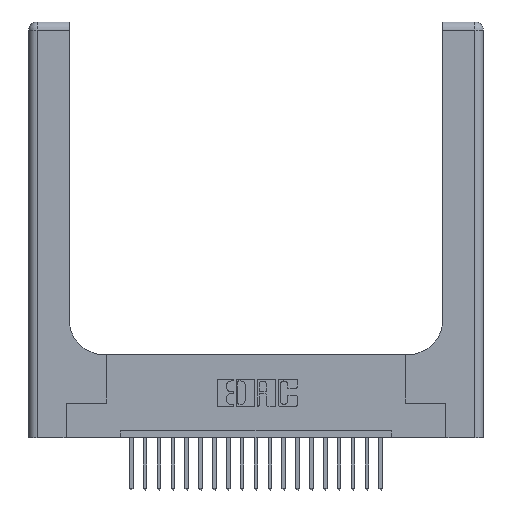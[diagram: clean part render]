
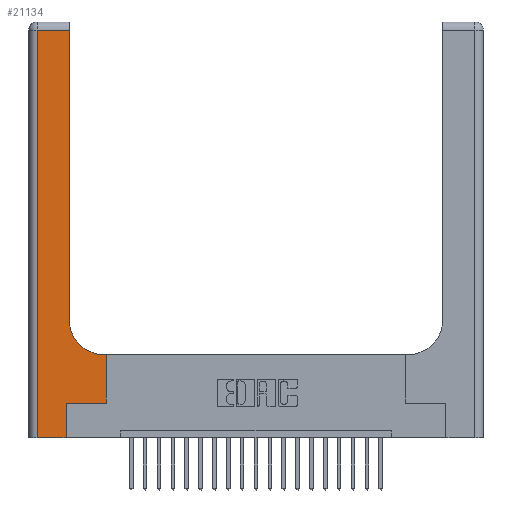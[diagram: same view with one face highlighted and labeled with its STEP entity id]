
A CAD part, top view. The second image highlights one B-rep face of the part: STEP entity #21134.
In plain terms, the highlighted planar face has unit normal (0, 0, 1).
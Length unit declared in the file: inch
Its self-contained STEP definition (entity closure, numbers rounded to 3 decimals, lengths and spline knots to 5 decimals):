
#349 = DIRECTION ( 'NONE',  ( 0., 1., 0. ) ) ;
#1554 = DIRECTION ( 'NONE',  ( 1., 0., 0. ) ) ;
#1664 = DIRECTION ( 'NONE',  ( 0., 0., -1. ) ) ;
#1735 = CARTESIAN_POINT ( 'NONE',  ( 0., 3., 0.37 ) ) ;
#2094 = LINE ( 'NONE', #3191, #18979 ) ;
#2331 = VERTEX_POINT ( 'NONE', #3034 ) ;
#2399 = DIRECTION ( 'NONE',  ( -1., 0., 0. ) ) ;
#2415 = CARTESIAN_POINT ( 'NONE',  ( 0.269, 0.25, 0.37 ) ) ;
#2566 = ORIENTED_EDGE ( 'NONE', *, *, #3840, .T. ) ;
#2600 = ORIENTED_EDGE ( 'NONE', *, *, #7431, .T. ) ;
#2825 = CARTESIAN_POINT ( 'NONE',  ( 0.5415, 0.6, 0.37 ) ) ;
#3034 = CARTESIAN_POINT ( 'NONE',  ( 0.5585, 0.25, 0.37 ) ) ;
#3191 = CARTESIAN_POINT ( 'NONE',  ( 0.5585, 0.25, 0.37 ) ) ;
#3840 = EDGE_CURVE ( 'NONE', #4231, #2331, #13804, .T. ) ;
#4231 = VERTEX_POINT ( 'NONE', #16587 ) ;
#4904 = DIRECTION ( 'NONE',  ( 0., -1., 0. ) ) ;
#4923 = VERTEX_POINT ( 'NONE', #15385 ) ;
#5019 = DIRECTION ( 'NONE',  ( -1., 0., 0. ) ) ;
#5157 = ORIENTED_EDGE ( 'NONE', *, *, #13256, .T. ) ;
#5191 = EDGE_LOOP ( 'NONE', ( #15216, #2600, #5157, #20965, #13100, #2566, #22404, #15001, #20932 ) ) ;
#6189 = LINE ( 'NONE', #8188, #12143 ) ;
#6477 = VECTOR ( 'NONE', #349, 39.37008 ) ;
#7431 = EDGE_CURVE ( 'NONE', #22213, #4923, #16874, .T. ) ;
#7611 = CARTESIAN_POINT ( 'NONE',  ( 0.2915, 0.6, 0.37 ) ) ;
#7626 = DIRECTION ( 'NONE',  ( 1., 0., 0. ) ) ;
#8188 = CARTESIAN_POINT ( 'NONE',  ( 0., 0., 0.37 ) ) ;
#8298 = CARTESIAN_POINT ( 'NONE',  ( 0.06, 3., 0.37 ) ) ;
#8425 = DIRECTION ( 'NONE',  ( 0., 1., 0. ) ) ;
#8561 = LINE ( 'NONE', #10622, #20061 ) ;
#8684 = CARTESIAN_POINT ( 'NONE',  ( 0.06, 0., 0.37 ) ) ;
#8877 = EDGE_CURVE ( 'NONE', #2331, #14995, #2094, .T. ) ;
#9233 = LINE ( 'NONE', #8298, #12751 ) ;
#9779 = CARTESIAN_POINT ( 'NONE',  ( 0.5415, 0.85, 0.37 ) ) ;
#9939 = VERTEX_POINT ( 'NONE', #11800 ) ;
#10622 = CARTESIAN_POINT ( 'NONE',  ( 0.2915, 3., 0.37 ) ) ;
#11289 = DIRECTION ( 'NONE',  ( 0., 0., -1. ) ) ;
#11800 = CARTESIAN_POINT ( 'NONE',  ( 0.2915, 0.85, 0.37 ) ) ;
#12143 = VECTOR ( 'NONE', #22107, 39.37008 ) ;
#12193 = CARTESIAN_POINT ( 'NONE',  ( 0.269, 0., 0.37 ) ) ;
#12751 = VECTOR ( 'NONE', #4904, 39.37008 ) ;
#12795 = CARTESIAN_POINT ( 'NONE',  ( 0., 2.94, 0.37 ) ) ;
#12851 = VECTOR ( 'NONE', #21375, 39.37008 ) ;
#13003 = VECTOR ( 'NONE', #7626, 39.37008 ) ;
#13100 = ORIENTED_EDGE ( 'NONE', *, *, #14706, .T. ) ;
#13256 = EDGE_CURVE ( 'NONE', #4923, #19142, #9233, .T. ) ;
#13804 = LINE ( 'NONE', #2415, #13003 ) ;
#14108 = VECTOR ( 'NONE', #2399, 39.37008 ) ;
#14439 = EDGE_CURVE ( 'NONE', #19142, #20180, #6189, .T. ) ;
#14706 = EDGE_CURVE ( 'NONE', #20180, #4231, #15707, .T. ) ;
#14995 = VERTEX_POINT ( 'NONE', #15081 ) ;
#15001 = ORIENTED_EDGE ( 'NONE', *, *, #19456, .T. ) ;
#15081 = CARTESIAN_POINT ( 'NONE',  ( 0.5585, 0.6, 0.37 ) ) ;
#15216 = ORIENTED_EDGE ( 'NONE', *, *, #16530, .T. ) ;
#15385 = CARTESIAN_POINT ( 'NONE',  ( 0.06, 2.94, 0.37 ) ) ;
#15707 = LINE ( 'NONE', #12193, #6477 ) ;
#16530 = EDGE_CURVE ( 'NONE', #9939, #22213, #8561, .T. ) ;
#16535 = AXIS2_PLACEMENT_3D ( 'NONE', #9779, #11289, #1554 ) ;
#16587 = CARTESIAN_POINT ( 'NONE',  ( 0.269, 0.25, 0.37 ) ) ;
#16874 = LINE ( 'NONE', #12795, #14108 ) ;
#16991 = AXIS2_PLACEMENT_3D ( 'NONE', #1735, #1664, #5019 ) ;
#17779 = CARTESIAN_POINT ( 'NONE',  ( 0.269, 0., 0.37 ) ) ;
#17805 = LINE ( 'NONE', #7611, #12851 ) ;
#17964 = CIRCLE ( 'NONE', #16535, 0.25 ) ;
#18937 = PLANE ( 'NONE',  #16991 ) ;
#18979 = VECTOR ( 'NONE', #8425, 39.37008 ) ;
#19142 = VERTEX_POINT ( 'NONE', #8684 ) ;
#19394 = DIRECTION ( 'NONE',  ( 0., 1., 0. ) ) ;
#19456 = EDGE_CURVE ( 'NONE', #14995, #19769, #17805, .T. ) ;
#19634 = FACE_OUTER_BOUND ( 'NONE', #5191, .T. ) ;
#19769 = VERTEX_POINT ( 'NONE', #2825 ) ;
#20061 = VECTOR ( 'NONE', #19394, 39.37008 ) ;
#20180 = VERTEX_POINT ( 'NONE', #17779 ) ;
#20932 = ORIENTED_EDGE ( 'NONE', *, *, #22456, .T. ) ;
#20965 = ORIENTED_EDGE ( 'NONE', *, *, #14439, .T. ) ;
#21134 = ADVANCED_FACE ( 'NONE', ( #19634 ), #18937, .F. ) ;
#21289 = CARTESIAN_POINT ( 'NONE',  ( 0.2915, 2.94, 0.37 ) ) ;
#21375 = DIRECTION ( 'NONE',  ( -1., 0., 0. ) ) ;
#22107 = DIRECTION ( 'NONE',  ( 1., 0., 0. ) ) ;
#22213 = VERTEX_POINT ( 'NONE', #21289 ) ;
#22404 = ORIENTED_EDGE ( 'NONE', *, *, #8877, .T. ) ;
#22456 = EDGE_CURVE ( 'NONE', #19769, #9939, #17964, .T. ) ;
